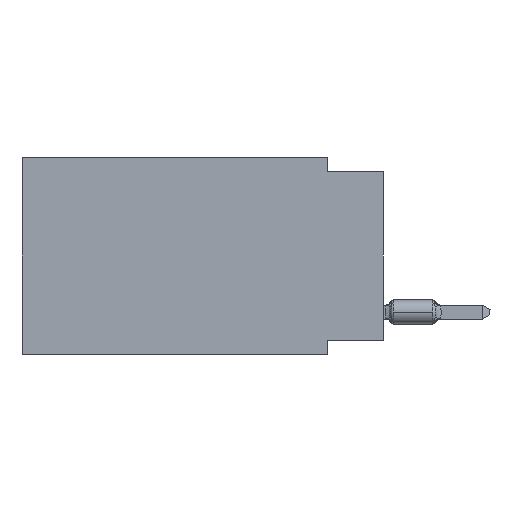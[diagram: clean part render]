
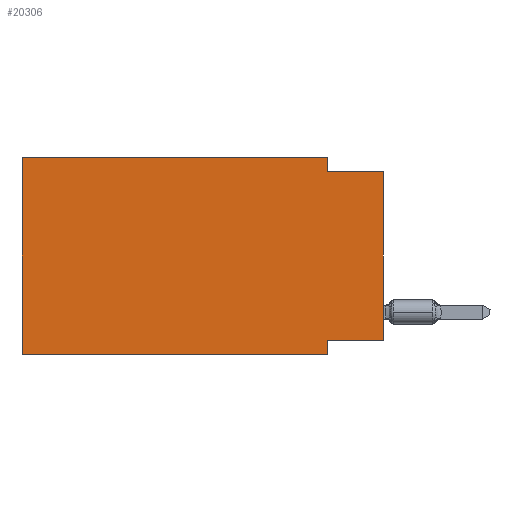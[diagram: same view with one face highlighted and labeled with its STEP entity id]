
A CAD part, left-side view. The second image highlights one B-rep face of the part: STEP entity #20306.
In plain terms, the highlighted planar face has unit normal (-1, 0, 0).
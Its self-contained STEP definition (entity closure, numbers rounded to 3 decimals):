
#689 = DIRECTION ( 'NONE',  ( 0., 0., -1. ) ) ;
#807 = DIRECTION ( 'NONE',  ( 1., 0., 0. ) ) ;
#1170 = LINE ( 'NONE', #20446, #12991 ) ;
#1384 = VERTEX_POINT ( 'NONE', #16741 ) ;
#1830 = EDGE_CURVE ( 'NONE', #11496, #19290, #1170, .T. ) ;
#1944 = LINE ( 'NONE', #16603, #3295 ) ;
#2041 = DIRECTION ( 'NONE',  ( 0., -1., 0. ) ) ;
#2295 = ORIENTED_EDGE ( 'NONE', *, *, #13951, .T. ) ;
#2515 = CARTESIAN_POINT ( 'NONE',  ( 0., 0., -0.635 ) ) ;
#2855 = CARTESIAN_POINT ( 'NONE',  ( 0., 2.54, 0. ) ) ;
#2884 = VECTOR ( 'NONE', #2041, 1000. ) ;
#3207 = VECTOR ( 'NONE', #21989, 1000. ) ;
#3295 = VECTOR ( 'NONE', #27995, 1000. ) ;
#3309 = LINE ( 'NONE', #14610, #3207 ) ;
#3806 = LINE ( 'NONE', #15696, #25844 ) ;
#3990 = DIRECTION ( 'NONE',  ( 0., 0., -1. ) ) ;
#4486 = LINE ( 'NONE', #28225, #26250 ) ;
#4875 = VERTEX_POINT ( 'NONE', #8580 ) ;
#5448 = CARTESIAN_POINT ( 'NONE',  ( 0., 16.383, 0. ) ) ;
#5673 = EDGE_CURVE ( 'NONE', #18204, #4875, #27942, .T. ) ;
#5737 = CARTESIAN_POINT ( 'NONE',  ( 0., 0., -8.255 ) ) ;
#8580 = CARTESIAN_POINT ( 'NONE',  ( 0., 2.54, 0. ) ) ;
#8965 = VECTOR ( 'NONE', #3990, 1000. ) ;
#9209 = EDGE_CURVE ( 'NONE', #19290, #1384, #26825, .T. ) ;
#9623 = CARTESIAN_POINT ( 'NONE',  ( 0., 16.383, 0. ) ) ;
#9641 = PLANE ( 'NONE',  #30393 ) ;
#10156 = EDGE_CURVE ( 'NONE', #20333, #28679, #4486, .T. ) ;
#10237 = DIRECTION ( 'NONE',  ( 0., 0., -1. ) ) ;
#10848 = EDGE_LOOP ( 'NONE', ( #2295, #26395, #24378, #19978, #23074, #11567, #28937, #19403 ) ) ;
#11496 = VERTEX_POINT ( 'NONE', #5737 ) ;
#11567 = ORIENTED_EDGE ( 'NONE', *, *, #19729, .T. ) ;
#11602 = CARTESIAN_POINT ( 'NONE',  ( 0., 16.383, 0. ) ) ;
#12991 = VECTOR ( 'NONE', #15366, 1000. ) ;
#13951 = EDGE_CURVE ( 'NONE', #11496, #28679, #3806, .T. ) ;
#14125 = EDGE_CURVE ( 'NONE', #20344, #18204, #3309, .T. ) ;
#14610 = CARTESIAN_POINT ( 'NONE',  ( 0., 16.383, 0. ) ) ;
#15366 = DIRECTION ( 'NONE',  ( 0., 1., 0. ) ) ;
#15696 = CARTESIAN_POINT ( 'NONE',  ( 0., 0., 0. ) ) ;
#16314 = EDGE_CURVE ( 'NONE', #4875, #20333, #23987, .T. ) ;
#16603 = CARTESIAN_POINT ( 'NONE',  ( 0., 16.383, -8.89 ) ) ;
#16741 = CARTESIAN_POINT ( 'NONE',  ( 0., 2.54, -8.89 ) ) ;
#17009 = CARTESIAN_POINT ( 'NONE',  ( 0., 2.54, -0.635 ) ) ;
#18204 = VERTEX_POINT ( 'NONE', #11602 ) ;
#19290 = VERTEX_POINT ( 'NONE', #24300 ) ;
#19403 = ORIENTED_EDGE ( 'NONE', *, *, #1830, .F. ) ;
#19605 = VECTOR ( 'NONE', #689, 1000. ) ;
#19729 = EDGE_CURVE ( 'NONE', #20344, #1384, #1944, .T. ) ;
#19978 = ORIENTED_EDGE ( 'NONE', *, *, #5673, .F. ) ;
#20306 = ADVANCED_FACE ( 'NONE', ( #21939 ), #9641, .F. ) ;
#20333 = VERTEX_POINT ( 'NONE', #17009 ) ;
#20344 = VERTEX_POINT ( 'NONE', #24397 ) ;
#20446 = CARTESIAN_POINT ( 'NONE',  ( 0., 0., -8.255 ) ) ;
#21939 = FACE_OUTER_BOUND ( 'NONE', #10848, .T. ) ;
#21989 = DIRECTION ( 'NONE',  ( 0., 0., 1. ) ) ;
#22646 = DIRECTION ( 'NONE',  ( 0., 0., 1. ) ) ;
#23074 = ORIENTED_EDGE ( 'NONE', *, *, #14125, .F. ) ;
#23987 = LINE ( 'NONE', #2855, #19605 ) ;
#24300 = CARTESIAN_POINT ( 'NONE',  ( 0., 2.54, -8.255 ) ) ;
#24378 = ORIENTED_EDGE ( 'NONE', *, *, #16314, .F. ) ;
#24397 = CARTESIAN_POINT ( 'NONE',  ( 0., 16.383, -8.89 ) ) ;
#25469 = DIRECTION ( 'NONE',  ( 0., -1., 0. ) ) ;
#25844 = VECTOR ( 'NONE', #22646, 1000. ) ;
#26250 = VECTOR ( 'NONE', #25469, 1000. ) ;
#26395 = ORIENTED_EDGE ( 'NONE', *, *, #10156, .F. ) ;
#26825 = LINE ( 'NONE', #27280, #8965 ) ;
#27280 = CARTESIAN_POINT ( 'NONE',  ( 0., 2.54, -8.89 ) ) ;
#27942 = LINE ( 'NONE', #9623, #2884 ) ;
#27995 = DIRECTION ( 'NONE',  ( 0., -1., 0. ) ) ;
#28225 = CARTESIAN_POINT ( 'NONE',  ( 0., 0., -0.635 ) ) ;
#28679 = VERTEX_POINT ( 'NONE', #2515 ) ;
#28937 = ORIENTED_EDGE ( 'NONE', *, *, #9209, .F. ) ;
#30393 = AXIS2_PLACEMENT_3D ( 'NONE', #5448, #807, #10237 ) ;
